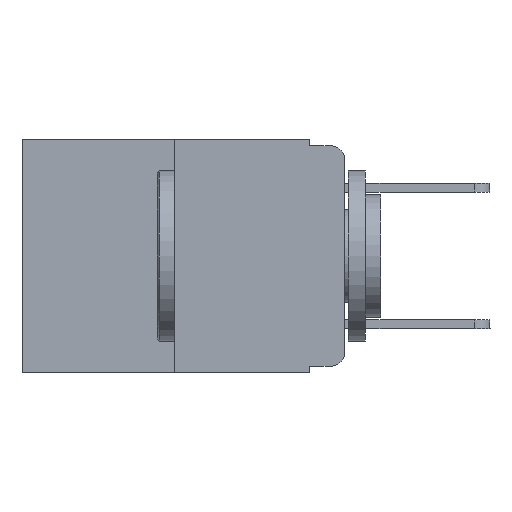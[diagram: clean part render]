
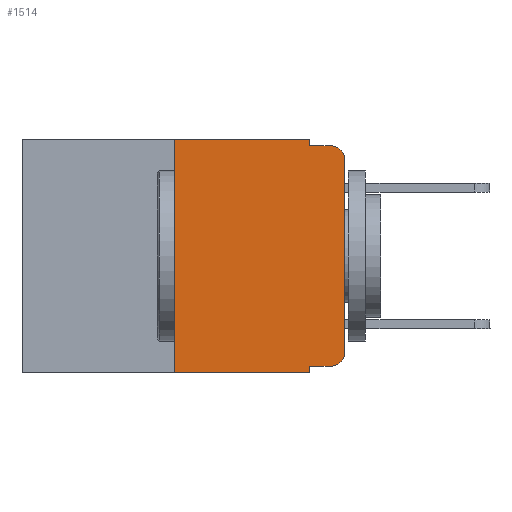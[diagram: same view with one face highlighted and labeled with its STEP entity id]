
A CAD part, left-side view. The second image highlights one B-rep face of the part: STEP entity #1514.
In plain terms, the highlighted planar face has unit normal (-1, 0, 0).
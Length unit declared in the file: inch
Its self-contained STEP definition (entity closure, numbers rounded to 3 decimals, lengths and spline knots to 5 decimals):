
#2 = CARTESIAN_POINT ( 'NONE',  ( 0., 0.473, 0. ) ) ;
#502 = DIRECTION ( 'NONE',  ( 0., -1., 0. ) ) ;
#531 = LINE ( 'NONE', #4183, #2593 ) ;
#768 = EDGE_CURVE ( 'NONE', #6149, #3558, #15003, .T. ) ;
#998 = DIRECTION ( 'NONE',  ( 0., 0., -1. ) ) ;
#1037 = EDGE_CURVE ( 'NONE', #14454, #11580, #1418, .T. ) ;
#1247 = DIRECTION ( 'NONE',  ( 0., 0., -1. ) ) ;
#1263 = DIRECTION ( 'NONE',  ( 0., -1., 0. ) ) ;
#1296 = LINE ( 'NONE', #11066, #12349 ) ;
#1300 = CARTESIAN_POINT ( 'NONE',  ( 0., 0.051, -0.333 ) ) ;
#1418 = LINE ( 'NONE', #9706, #3047 ) ;
#1420 = VERTEX_POINT ( 'NONE', #3201 ) ;
#1514 = ADVANCED_FACE ( 'NONE', ( #2273 ), #10853, .F. ) ;
#1664 = CARTESIAN_POINT ( 'NONE',  ( 0., 0.051, -0.01 ) ) ;
#1895 = EDGE_CURVE ( 'NONE', #2051, #14454, #7306, .T. ) ;
#2003 = VERTEX_POINT ( 'NONE', #1300 ) ;
#2051 = VERTEX_POINT ( 'NONE', #6372 ) ;
#2260 = CIRCLE ( 'NONE', #3996, 0.02 ) ;
#2273 = FACE_OUTER_BOUND ( 'NONE', #2553, .T. ) ;
#2277 = EDGE_CURVE ( 'NONE', #2003, #1420, #6600, .T. ) ;
#2440 = ORIENTED_EDGE ( 'NONE', *, *, #2277, .T. ) ;
#2553 = EDGE_LOOP ( 'NONE', ( #3249, #9380, #7402, #9194, #11529, #10479, #15244, #3989, #2440, #13097 ) ) ;
#2593 = VECTOR ( 'NONE', #3027, 39.37008 ) ;
#2631 = DIRECTION ( 'NONE',  ( 0., -1., 0. ) ) ;
#3027 = DIRECTION ( 'NONE',  ( 0., 0., -1. ) ) ;
#3047 = VECTOR ( 'NONE', #1263, 39.37008 ) ;
#3201 = CARTESIAN_POINT ( 'NONE',  ( 0., 0.02, -0.333 ) ) ;
#3249 = ORIENTED_EDGE ( 'NONE', *, *, #11767, .T. ) ;
#3323 = VECTOR ( 'NONE', #3491, 39.37008 ) ;
#3410 = CARTESIAN_POINT ( 'NONE',  ( 0., 0.051, -0.01 ) ) ;
#3426 = EDGE_CURVE ( 'NONE', #2003, #11301, #531, .T. ) ;
#3491 = DIRECTION ( 'NONE',  ( 0., 0., 1. ) ) ;
#3558 = VERTEX_POINT ( 'NONE', #15030 ) ;
#3989 = ORIENTED_EDGE ( 'NONE', *, *, #3426, .F. ) ;
#3996 = AXIS2_PLACEMENT_3D ( 'NONE', #4588, #11710, #998 ) ;
#4183 = CARTESIAN_POINT ( 'NONE',  ( 0., 0.051, 0. ) ) ;
#4205 = VERTEX_POINT ( 'NONE', #13439 ) ;
#4588 = CARTESIAN_POINT ( 'NONE',  ( 0., 0.02, -0.03 ) ) ;
#5042 = EDGE_CURVE ( 'NONE', #2051, #11301, #1296, .T. ) ;
#6149 = VERTEX_POINT ( 'NONE', #3410 ) ;
#6169 = EDGE_CURVE ( 'NONE', #11580, #6149, #12007, .T. ) ;
#6372 = CARTESIAN_POINT ( 'NONE',  ( 0., 0.25, -0.343 ) ) ;
#6600 = LINE ( 'NONE', #12611, #7076 ) ;
#6625 = CARTESIAN_POINT ( 'NONE',  ( 0., 0., -0.03 ) ) ;
#7076 = VECTOR ( 'NONE', #11378, 39.37008 ) ;
#7156 = VECTOR ( 'NONE', #502, 39.37008 ) ;
#7306 = LINE ( 'NONE', #14411, #3323 ) ;
#7402 = ORIENTED_EDGE ( 'NONE', *, *, #768, .F. ) ;
#8098 = CARTESIAN_POINT ( 'NONE',  ( 0., 0.051, 0. ) ) ;
#8475 = CIRCLE ( 'NONE', #13963, 0.02 ) ;
#8773 = AXIS2_PLACEMENT_3D ( 'NONE', #2, #9522, #1247 ) ;
#8907 = CARTESIAN_POINT ( 'NONE',  ( 0., 0.051, 0. ) ) ;
#9194 = ORIENTED_EDGE ( 'NONE', *, *, #6169, .F. ) ;
#9204 = DIRECTION ( 'NONE',  ( 0., 0., -1. ) ) ;
#9380 = ORIENTED_EDGE ( 'NONE', *, *, #12226, .T. ) ;
#9417 = DIRECTION ( 'NONE',  ( 0., 0., -1. ) ) ;
#9522 = DIRECTION ( 'NONE',  ( 1., 0., 0. ) ) ;
#9706 = CARTESIAN_POINT ( 'NONE',  ( 0., 0.473, 0. ) ) ;
#10479 = ORIENTED_EDGE ( 'NONE', *, *, #1895, .F. ) ;
#10549 = LINE ( 'NONE', #14059, #14709 ) ;
#10853 = PLANE ( 'NONE',  #8773 ) ;
#11066 = CARTESIAN_POINT ( 'NONE',  ( 0., 0.473, -0.343 ) ) ;
#11301 = VERTEX_POINT ( 'NONE', #15238 ) ;
#11378 = DIRECTION ( 'NONE',  ( 0., -1., 0. ) ) ;
#11529 = ORIENTED_EDGE ( 'NONE', *, *, #1037, .F. ) ;
#11580 = VERTEX_POINT ( 'NONE', #8907 ) ;
#11710 = DIRECTION ( 'NONE',  ( -1., 0., 0. ) ) ;
#11713 = EDGE_CURVE ( 'NONE', #1420, #4205, #8475, .T. ) ;
#11767 = EDGE_CURVE ( 'NONE', #4205, #12097, #10549, .T. ) ;
#11797 = DIRECTION ( 'NONE',  ( 0., 0., 1. ) ) ;
#12007 = LINE ( 'NONE', #8098, #12864 ) ;
#12097 = VERTEX_POINT ( 'NONE', #6625 ) ;
#12226 = EDGE_CURVE ( 'NONE', #12097, #3558, #2260, .T. ) ;
#12349 = VECTOR ( 'NONE', #2631, 39.37008 ) ;
#12611 = CARTESIAN_POINT ( 'NONE',  ( 0., 0.051, -0.333 ) ) ;
#12864 = VECTOR ( 'NONE', #9417, 39.37008 ) ;
#13037 = DIRECTION ( 'NONE',  ( -1., 0., 0. ) ) ;
#13097 = ORIENTED_EDGE ( 'NONE', *, *, #11713, .T. ) ;
#13439 = CARTESIAN_POINT ( 'NONE',  ( 0., 0., -0.313 ) ) ;
#13895 = CARTESIAN_POINT ( 'NONE',  ( 0., 0.02, -0.313 ) ) ;
#13963 = AXIS2_PLACEMENT_3D ( 'NONE', #13895, #13037, #9204 ) ;
#14059 = CARTESIAN_POINT ( 'NONE',  ( 0., 0., 0. ) ) ;
#14411 = CARTESIAN_POINT ( 'NONE',  ( 0., 0.25, 0. ) ) ;
#14454 = VERTEX_POINT ( 'NONE', #15093 ) ;
#14709 = VECTOR ( 'NONE', #11797, 39.37008 ) ;
#15003 = LINE ( 'NONE', #1664, #7156 ) ;
#15030 = CARTESIAN_POINT ( 'NONE',  ( 0., 0.02, -0.01 ) ) ;
#15093 = CARTESIAN_POINT ( 'NONE',  ( 0., 0.25, 0. ) ) ;
#15238 = CARTESIAN_POINT ( 'NONE',  ( 0., 0.051, -0.343 ) ) ;
#15244 = ORIENTED_EDGE ( 'NONE', *, *, #5042, .T. ) ;
